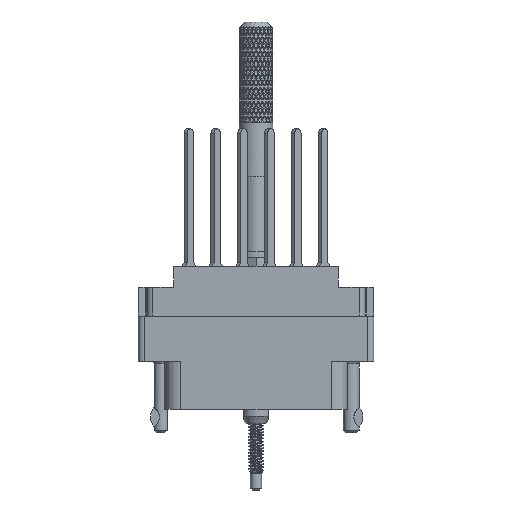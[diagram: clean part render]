
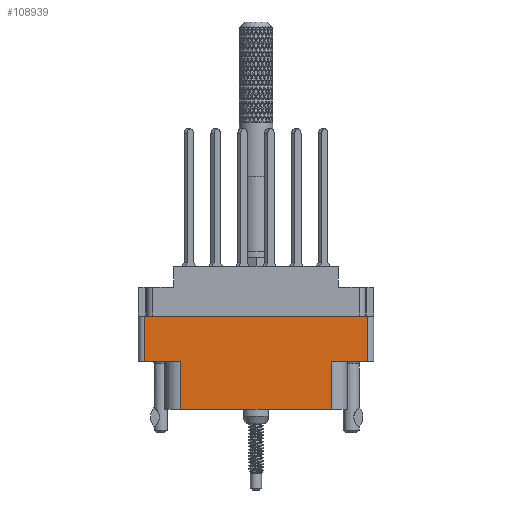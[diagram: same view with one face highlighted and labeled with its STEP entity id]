
A CAD part, front view. The second image highlights one B-rep face of the part: STEP entity #108939.
In plain terms, the highlighted planar face has unit normal (0, -1, 0).
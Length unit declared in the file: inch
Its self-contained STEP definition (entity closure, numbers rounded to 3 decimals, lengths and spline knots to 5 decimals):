
#3068 = CARTESIAN_POINT ( 'NONE',  ( 0.624, -0.343, -0.277 ) ) ;
#8577 = LINE ( 'NONE', #68244, #92537 ) ;
#12818 = CARTESIAN_POINT ( 'NONE',  ( -0.42, -0.343, -0.798 ) ) ;
#13598 = DIRECTION ( 'NONE',  ( 1., 0., 0. ) ) ;
#13627 = DIRECTION ( 'NONE',  ( 1., 0., 0. ) ) ;
#18322 = LINE ( 'NONE', #71020, #74249 ) ;
#20262 = CARTESIAN_POINT ( 'NONE',  ( 0.42, -0.343, -0.798 ) ) ;
#20357 = VERTEX_POINT ( 'NONE', #31570 ) ;
#23679 = CARTESIAN_POINT ( 'NONE',  ( 0., -0.343, -0.529 ) ) ;
#26946 = ORIENTED_EDGE ( 'NONE', *, *, #98283, .T. ) ;
#27492 = DIRECTION ( 'NONE',  ( 0., 0., -1. ) ) ;
#28248 = VERTEX_POINT ( 'NONE', #12818 ) ;
#31570 = CARTESIAN_POINT ( 'NONE',  ( 0.42, -0.343, -0.529 ) ) ;
#35907 = VECTOR ( 'NONE', #133804, 39.37008 ) ;
#36066 = VERTEX_POINT ( 'NONE', #20262 ) ;
#38660 = DIRECTION ( 'NONE',  ( -1., 0., 0. ) ) ;
#40700 = ORIENTED_EDGE ( 'NONE', *, *, #117455, .F. ) ;
#42517 = LINE ( 'NONE', #132117, #180046 ) ;
#46861 = ORIENTED_EDGE ( 'NONE', *, *, #114473, .F. ) ;
#49098 = ORIENTED_EDGE ( 'NONE', *, *, #66051, .F. ) ;
#55237 = LINE ( 'NONE', #175409, #104244 ) ;
#58631 = CARTESIAN_POINT ( 'NONE',  ( -0.656, -0.343, -0.277 ) ) ;
#58923 = CARTESIAN_POINT ( 'NONE',  ( -0.624, -0.343, -0.798 ) ) ;
#60248 = VERTEX_POINT ( 'NONE', #70955 ) ;
#60978 = VECTOR ( 'NONE', #121506, 39.37008 ) ;
#66051 = EDGE_CURVE ( 'NONE', #20357, #36066, #55237, .T. ) ;
#68244 = CARTESIAN_POINT ( 'NONE',  ( -0.624, -0.343, -0.798 ) ) ;
#70955 = CARTESIAN_POINT ( 'NONE',  ( -0.624, -0.343, -0.529 ) ) ;
#71020 = CARTESIAN_POINT ( 'NONE',  ( -0.42, -0.343, -0.529 ) ) ;
#72614 = DIRECTION ( 'NONE',  ( 0., -1., 0. ) ) ;
#74249 = VECTOR ( 'NONE', #176478, 39.37008 ) ;
#74523 = PLANE ( 'NONE',  #192055 ) ;
#76163 = VERTEX_POINT ( 'NONE', #147442 ) ;
#89140 = EDGE_CURVE ( 'NONE', #60248, #139964, #42517, .T. ) ;
#91737 = VECTOR ( 'NONE', #13627, 39.37008 ) ;
#92537 = VECTOR ( 'NONE', #113741, 39.37008 ) ;
#98283 = EDGE_CURVE ( 'NONE', #139964, #28248, #18322, .T. ) ;
#100530 = LINE ( 'NONE', #167103, #60978 ) ;
#101044 = VERTEX_POINT ( 'NONE', #3068 ) ;
#103306 = EDGE_LOOP ( 'NONE', ( #26946, #121224, #49098, #40700, #128604, #46861, #133479, #104390 ) ) ;
#104244 = VECTOR ( 'NONE', #27492, 39.37008 ) ;
#104390 = ORIENTED_EDGE ( 'NONE', *, *, #89140, .T. ) ;
#108372 = VERTEX_POINT ( 'NONE', #166958 ) ;
#108939 = ADVANCED_FACE ( 'NONE', ( #162958 ), #74523, .T. ) ;
#111584 = EDGE_CURVE ( 'NONE', #28248, #36066, #185077, .T. ) ;
#113741 = DIRECTION ( 'NONE',  ( 0., 0., 1. ) ) ;
#114473 = EDGE_CURVE ( 'NONE', #108372, #101044, #150002, .T. ) ;
#117455 = EDGE_CURVE ( 'NONE', #76163, #20357, #168136, .T. ) ;
#118160 = CARTESIAN_POINT ( 'NONE',  ( -0.624, -0.343, -0.798 ) ) ;
#121224 = ORIENTED_EDGE ( 'NONE', *, *, #111584, .T. ) ;
#121506 = DIRECTION ( 'NONE',  ( 0., 0., 1. ) ) ;
#128604 = ORIENTED_EDGE ( 'NONE', *, *, #188683, .T. ) ;
#132117 = CARTESIAN_POINT ( 'NONE',  ( 0., -0.343, -0.529 ) ) ;
#133479 = ORIENTED_EDGE ( 'NONE', *, *, #166618, .F. ) ;
#133737 = DIRECTION ( 'NONE',  ( 0., 0., -1. ) ) ;
#133804 = DIRECTION ( 'NONE',  ( 1., 0., 0. ) ) ;
#139964 = VERTEX_POINT ( 'NONE', #183743 ) ;
#147442 = CARTESIAN_POINT ( 'NONE',  ( 0.624, -0.343, -0.529 ) ) ;
#150002 = LINE ( 'NONE', #58631, #91737 ) ;
#162958 = FACE_OUTER_BOUND ( 'NONE', #103306, .T. ) ;
#166618 = EDGE_CURVE ( 'NONE', #60248, #108372, #8577, .T. ) ;
#166958 = CARTESIAN_POINT ( 'NONE',  ( -0.624, -0.343, -0.277 ) ) ;
#167103 = CARTESIAN_POINT ( 'NONE',  ( 0.624, -0.343, -0.798 ) ) ;
#168136 = LINE ( 'NONE', #23679, #184385 ) ;
#175409 = CARTESIAN_POINT ( 'NONE',  ( 0.42, -0.343, -0.529 ) ) ;
#176478 = DIRECTION ( 'NONE',  ( 0., 0., -1. ) ) ;
#180046 = VECTOR ( 'NONE', #13598, 39.37008 ) ;
#183743 = CARTESIAN_POINT ( 'NONE',  ( -0.42, -0.343, -0.529 ) ) ;
#184385 = VECTOR ( 'NONE', #38660, 39.37008 ) ;
#185077 = LINE ( 'NONE', #118160, #35907 ) ;
#188683 = EDGE_CURVE ( 'NONE', #76163, #101044, #100530, .T. ) ;
#192055 = AXIS2_PLACEMENT_3D ( 'NONE', #58923, #72614, #133737 ) ;
